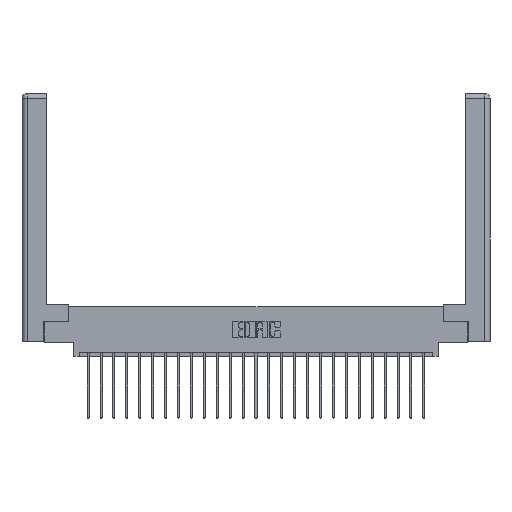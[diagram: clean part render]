
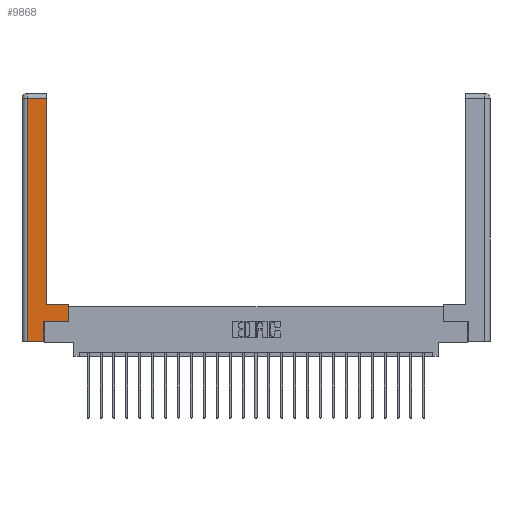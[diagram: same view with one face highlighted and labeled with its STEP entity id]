
A CAD part, top view. The second image highlights one B-rep face of the part: STEP entity #9868.
In plain terms, the highlighted planar face has unit normal (0, 0, 1).
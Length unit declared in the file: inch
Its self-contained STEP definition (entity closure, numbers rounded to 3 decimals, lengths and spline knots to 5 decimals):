
#118 = ORIENTED_EDGE ( 'NONE', *, *, #18202, .T. ) ;
#721 = CARTESIAN_POINT ( 'NONE',  ( 0.0615, 2.94, 0. ) ) ;
#912 = EDGE_CURVE ( 'NONE', #3585, #10762, #8303, .T. ) ;
#2696 = VECTOR ( 'NONE', #4527, 39.37008 ) ;
#2704 = EDGE_CURVE ( 'NONE', #10762, #14057, #9641, .T. ) ;
#3585 = VERTEX_POINT ( 'NONE', #25083 ) ;
#4360 = CARTESIAN_POINT ( 'NONE',  ( 0.295, 2.94, 0. ) ) ;
#4527 = DIRECTION ( 'NONE',  ( -1., 0., 0. ) ) ;
#4686 = DIRECTION ( 'NONE',  ( 0., 1., 0. ) ) ;
#5118 = VECTOR ( 'NONE', #5212, 39.37008 ) ;
#5208 = DIRECTION ( 'NONE',  ( -1., 0., 0. ) ) ;
#5212 = DIRECTION ( 'NONE',  ( 1., 0., 0. ) ) ;
#5303 = EDGE_CURVE ( 'NONE', #14057, #16822, #11662, .T. ) ;
#5600 = ORIENTED_EDGE ( 'NONE', *, *, #15744, .T. ) ;
#5627 = DIRECTION ( 'NONE',  ( 0., -1., 0. ) ) ;
#7047 = VECTOR ( 'NONE', #9134, 39.37008 ) ;
#7237 = VECTOR ( 'NONE', #5627, 39.37008 ) ;
#7738 = VERTEX_POINT ( 'NONE', #14002 ) ;
#8303 = LINE ( 'NONE', #16542, #12638 ) ;
#9134 = DIRECTION ( 'NONE',  ( -1., 0., 0. ) ) ;
#9247 = VERTEX_POINT ( 'NONE', #23363 ) ;
#9641 = LINE ( 'NONE', #17111, #13639 ) ;
#9868 = ADVANCED_FACE ( 'NONE', ( #24134 ), #18874, .F. ) ;
#10012 = ORIENTED_EDGE ( 'NONE', *, *, #10676, .T. ) ;
#10295 = VECTOR ( 'NONE', #4686, 39.37008 ) ;
#10676 = EDGE_CURVE ( 'NONE', #16822, #9247, #16331, .T. ) ;
#10755 = VECTOR ( 'NONE', #18246, 39.37008 ) ;
#10762 = VERTEX_POINT ( 'NONE', #22964 ) ;
#11389 = CARTESIAN_POINT ( 'NONE',  ( 0.565, 0.45, 0. ) ) ;
#11396 = ORIENTED_EDGE ( 'NONE', *, *, #912, .T. ) ;
#11662 = LINE ( 'NONE', #22301, #10755 ) ;
#11892 = ORIENTED_EDGE ( 'NONE', *, *, #20544, .T. ) ;
#12638 = VECTOR ( 'NONE', #20542, 39.37008 ) ;
#12711 = VERTEX_POINT ( 'NONE', #721 ) ;
#13024 = CARTESIAN_POINT ( 'NONE',  ( 0.265, 0., 0. ) ) ;
#13055 = ORIENTED_EDGE ( 'NONE', *, *, #2704, .T. ) ;
#13112 = CARTESIAN_POINT ( 'NONE',  ( 0., 0., 0. ) ) ;
#13639 = VECTOR ( 'NONE', #14955, 39.37008 ) ;
#14002 = CARTESIAN_POINT ( 'NONE',  ( 0.0615, 0., 0. ) ) ;
#14057 = VERTEX_POINT ( 'NONE', #23461 ) ;
#14656 = CARTESIAN_POINT ( 'NONE',  ( 0.295, 3., 0. ) ) ;
#14955 = DIRECTION ( 'NONE',  ( 1., 0., 0. ) ) ;
#15744 = EDGE_CURVE ( 'NONE', #9247, #17023, #23940, .T. ) ;
#15973 = LINE ( 'NONE', #13024, #5118 ) ;
#16174 = ORIENTED_EDGE ( 'NONE', *, *, #5303, .T. ) ;
#16331 = LINE ( 'NONE', #16380, #2696 ) ;
#16380 = CARTESIAN_POINT ( 'NONE',  ( 0.295, 0.45, 0. ) ) ;
#16542 = CARTESIAN_POINT ( 'NONE',  ( 0.265, 0.245, 0. ) ) ;
#16774 = CARTESIAN_POINT ( 'NONE',  ( 0.0615, 2.94, 0. ) ) ;
#16822 = VERTEX_POINT ( 'NONE', #11389 ) ;
#17023 = VERTEX_POINT ( 'NONE', #4360 ) ;
#17111 = CARTESIAN_POINT ( 'NONE',  ( 0.565, 0.245, 0. ) ) ;
#17538 = CARTESIAN_POINT ( 'NONE',  ( 0.0615, 0., 0. ) ) ;
#17803 = LINE ( 'NONE', #17538, #7237 ) ;
#18202 = EDGE_CURVE ( 'NONE', #17023, #12711, #20409, .T. ) ;
#18246 = DIRECTION ( 'NONE',  ( 0., 1., 0. ) ) ;
#18874 = PLANE ( 'NONE',  #22290 ) ;
#19493 = ORIENTED_EDGE ( 'NONE', *, *, #20655, .T. ) ;
#20409 = LINE ( 'NONE', #16774, #7047 ) ;
#20542 = DIRECTION ( 'NONE',  ( 0., 1., 0. ) ) ;
#20544 = EDGE_CURVE ( 'NONE', #7738, #3585, #15973, .T. ) ;
#20573 = EDGE_LOOP ( 'NONE', ( #5600, #118, #19493, #11892, #11396, #13055, #16174, #10012 ) ) ;
#20655 = EDGE_CURVE ( 'NONE', #12711, #7738, #17803, .T. ) ;
#22290 = AXIS2_PLACEMENT_3D ( 'NONE', #13112, #22751, #5208 ) ;
#22301 = CARTESIAN_POINT ( 'NONE',  ( 0.565, 0.45, 0. ) ) ;
#22751 = DIRECTION ( 'NONE',  ( 0., 0., -1. ) ) ;
#22964 = CARTESIAN_POINT ( 'NONE',  ( 0.265, 0.245, 0. ) ) ;
#23363 = CARTESIAN_POINT ( 'NONE',  ( 0.295, 0.45, 0. ) ) ;
#23461 = CARTESIAN_POINT ( 'NONE',  ( 0.565, 0.245, 0. ) ) ;
#23940 = LINE ( 'NONE', #14656, #10295 ) ;
#24134 = FACE_OUTER_BOUND ( 'NONE', #20573, .T. ) ;
#25083 = CARTESIAN_POINT ( 'NONE',  ( 0.265, 0., 0. ) ) ;
